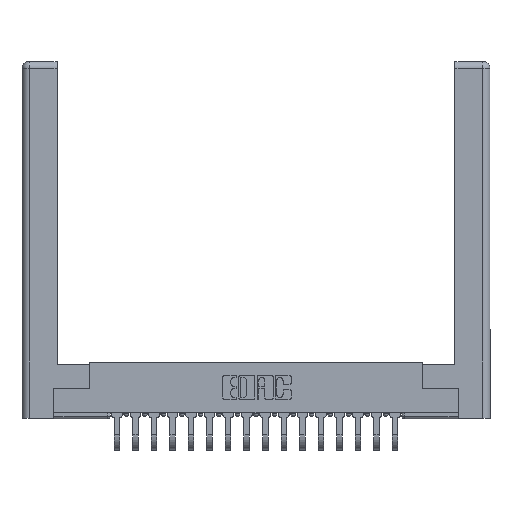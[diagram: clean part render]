
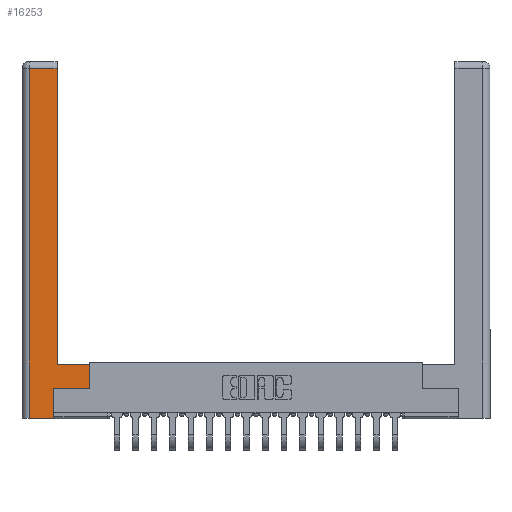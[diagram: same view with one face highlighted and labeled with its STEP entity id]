
A CAD part, top view. The second image highlights one B-rep face of the part: STEP entity #16253.
In plain terms, the highlighted planar face has unit normal (0, 0, 1).
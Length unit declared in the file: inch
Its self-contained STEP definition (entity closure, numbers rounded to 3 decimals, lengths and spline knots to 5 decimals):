
#89 = DIRECTION ( 'NONE',  ( 0., 1., 0. ) ) ;
#764 = CARTESIAN_POINT ( 'NONE',  ( 0.0615, 0., 0. ) ) ;
#1431 = CARTESIAN_POINT ( 'NONE',  ( 0., 0., 0. ) ) ;
#1544 = EDGE_LOOP ( 'NONE', ( #3499, #14270, #6038, #11706, #18570, #7941, #17949, #11851 ) ) ;
#1571 = CARTESIAN_POINT ( 'NONE',  ( 0.265, 0., 0. ) ) ;
#2581 = CARTESIAN_POINT ( 'NONE',  ( 0.265, 0.245, 0. ) ) ;
#2611 = EDGE_CURVE ( 'NONE', #13989, #8844, #4610, .T. ) ;
#2829 = DIRECTION ( 'NONE',  ( -1., 0., 0. ) ) ;
#3032 = EDGE_CURVE ( 'NONE', #11208, #5406, #19630, .T. ) ;
#3409 = CARTESIAN_POINT ( 'NONE',  ( 0.265, 0.245, 0. ) ) ;
#3498 = VECTOR ( 'NONE', #19659, 39.37008 ) ;
#3499 = ORIENTED_EDGE ( 'NONE', *, *, #14196, .T. ) ;
#3619 = VECTOR ( 'NONE', #89, 39.37008 ) ;
#3883 = VERTEX_POINT ( 'NONE', #8989 ) ;
#4610 = LINE ( 'NONE', #13573, #3498 ) ;
#4687 = DIRECTION ( 'NONE',  ( -1., 0., 0. ) ) ;
#5406 = VERTEX_POINT ( 'NONE', #11757 ) ;
#5838 = CARTESIAN_POINT ( 'NONE',  ( 0.0615, 0., 0. ) ) ;
#6038 = ORIENTED_EDGE ( 'NONE', *, *, #12766, .T. ) ;
#6352 = CARTESIAN_POINT ( 'NONE',  ( 0.295, 0.45, 0. ) ) ;
#6540 = DIRECTION ( 'NONE',  ( 0., -1., 0. ) ) ;
#6813 = VECTOR ( 'NONE', #18301, 39.37008 ) ;
#7417 = CARTESIAN_POINT ( 'NONE',  ( 0.265, 0., 0. ) ) ;
#7607 = CARTESIAN_POINT ( 'NONE',  ( 0.295, 0.45, 0. ) ) ;
#7685 = DIRECTION ( 'NONE',  ( 0., 0., -1. ) ) ;
#7847 = VERTEX_POINT ( 'NONE', #5838 ) ;
#7941 = ORIENTED_EDGE ( 'NONE', *, *, #2611, .T. ) ;
#8591 = VECTOR ( 'NONE', #4687, 39.37008 ) ;
#8844 = VERTEX_POINT ( 'NONE', #10011 ) ;
#8989 = CARTESIAN_POINT ( 'NONE',  ( 0.565, 0.45, 0. ) ) ;
#9225 = CARTESIAN_POINT ( 'NONE',  ( 0.295, 3., 0. ) ) ;
#9272 = FACE_OUTER_BOUND ( 'NONE', #1544, .T. ) ;
#10011 = CARTESIAN_POINT ( 'NONE',  ( 0.565, 0.245, 0. ) ) ;
#10722 = CARTESIAN_POINT ( 'NONE',  ( 0.565, 0.45, 0. ) ) ;
#11073 = LINE ( 'NONE', #7417, #16018 ) ;
#11208 = VERTEX_POINT ( 'NONE', #17216 ) ;
#11706 = ORIENTED_EDGE ( 'NONE', *, *, #14518, .T. ) ;
#11757 = CARTESIAN_POINT ( 'NONE',  ( 0.0615, 2.94, 0. ) ) ;
#11851 = ORIENTED_EDGE ( 'NONE', *, *, #11875, .T. ) ;
#11875 = EDGE_CURVE ( 'NONE', #3883, #12680, #18270, .T. ) ;
#11978 = DIRECTION ( 'NONE',  ( -1., 0., 0. ) ) ;
#12680 = VERTEX_POINT ( 'NONE', #6352 ) ;
#12766 = EDGE_CURVE ( 'NONE', #5406, #7847, #18792, .T. ) ;
#12864 = DIRECTION ( 'NONE',  ( 0., 1., 0. ) ) ;
#13473 = PLANE ( 'NONE',  #18599 ) ;
#13573 = CARTESIAN_POINT ( 'NONE',  ( 0.565, 0.245, 0. ) ) ;
#13714 = LINE ( 'NONE', #10722, #3619 ) ;
#13989 = VERTEX_POINT ( 'NONE', #2581 ) ;
#14196 = EDGE_CURVE ( 'NONE', #12680, #11208, #15404, .T. ) ;
#14270 = ORIENTED_EDGE ( 'NONE', *, *, #3032, .T. ) ;
#14518 = EDGE_CURVE ( 'NONE', #7847, #19145, #11073, .T. ) ;
#15177 = VECTOR ( 'NONE', #12864, 39.37008 ) ;
#15404 = LINE ( 'NONE', #9225, #6813 ) ;
#15417 = EDGE_CURVE ( 'NONE', #8844, #3883, #13714, .T. ) ;
#15966 = LINE ( 'NONE', #3409, #15177 ) ;
#16018 = VECTOR ( 'NONE', #17155, 39.37008 ) ;
#16253 = ADVANCED_FACE ( 'NONE', ( #9272 ), #13473, .F. ) ;
#16453 = CARTESIAN_POINT ( 'NONE',  ( 0.0615, 2.94, 0. ) ) ;
#16823 = VECTOR ( 'NONE', #11978, 39.37008 ) ;
#17155 = DIRECTION ( 'NONE',  ( 1., 0., 0. ) ) ;
#17216 = CARTESIAN_POINT ( 'NONE',  ( 0.295, 2.94, 0. ) ) ;
#17768 = VECTOR ( 'NONE', #6540, 39.37008 ) ;
#17949 = ORIENTED_EDGE ( 'NONE', *, *, #15417, .T. ) ;
#18270 = LINE ( 'NONE', #7607, #16823 ) ;
#18301 = DIRECTION ( 'NONE',  ( 0., 1., 0. ) ) ;
#18380 = EDGE_CURVE ( 'NONE', #19145, #13989, #15966, .T. ) ;
#18570 = ORIENTED_EDGE ( 'NONE', *, *, #18380, .T. ) ;
#18599 = AXIS2_PLACEMENT_3D ( 'NONE', #1431, #7685, #2829 ) ;
#18792 = LINE ( 'NONE', #764, #17768 ) ;
#19145 = VERTEX_POINT ( 'NONE', #1571 ) ;
#19630 = LINE ( 'NONE', #16453, #8591 ) ;
#19659 = DIRECTION ( 'NONE',  ( 1., 0., 0. ) ) ;
